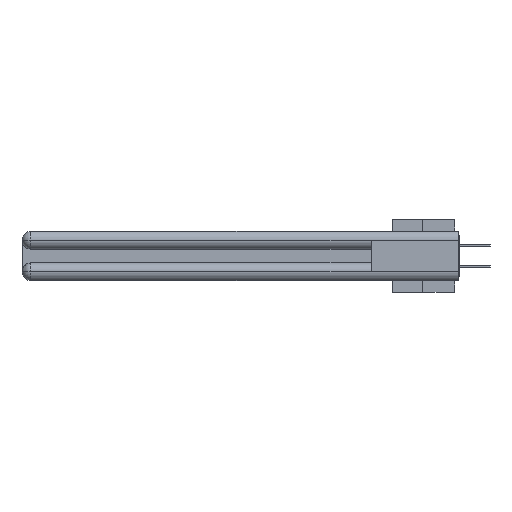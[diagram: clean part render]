
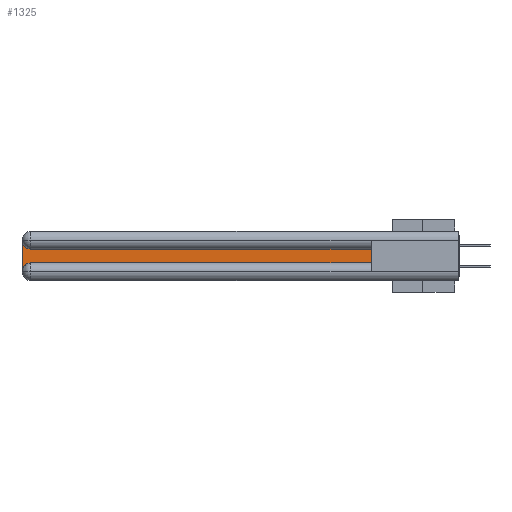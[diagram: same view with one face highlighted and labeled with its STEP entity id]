
A CAD part, left-side view. The second image highlights one B-rep face of the part: STEP entity #1325.
In plain terms, the highlighted planar face has unit normal (-1, 0, 0).
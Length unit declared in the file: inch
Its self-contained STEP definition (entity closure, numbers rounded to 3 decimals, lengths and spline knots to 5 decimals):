
#74 = VECTOR ( 'NONE', #16724, 39.37008 ) ;
#1325 = ADVANCED_FACE ( 'NONE', ( #25276 ), #7917, .F. ) ;
#1981 = LINE ( 'NONE', #8836, #11618 ) ;
#2189 = CARTESIAN_POINT ( 'NONE',  ( 0.075, 3., -0.1225 ) ) ;
#2423 = VECTOR ( 'NONE', #4829, 39.37008 ) ;
#2667 = EDGE_CURVE ( 'NONE', #15542, #8609, #1981, .T. ) ;
#4596 = CARTESIAN_POINT ( 'NONE',  ( 0.075, 3., -0.2775 ) ) ;
#4829 = DIRECTION ( 'NONE',  ( 0., 0., -1. ) ) ;
#6601 = EDGE_CURVE ( 'NONE', #27151, #16936, #23314, .T. ) ;
#7165 = DIRECTION ( 'NONE',  ( 0., 0., -1. ) ) ;
#7917 = PLANE ( 'NONE',  #29174 ) ;
#8261 = CARTESIAN_POINT ( 'NONE',  ( 0.075, 2.94, -0.1225 ) ) ;
#8609 = VERTEX_POINT ( 'NONE', #13999 ) ;
#8827 = VERTEX_POINT ( 'NONE', #4596 ) ;
#8836 = CARTESIAN_POINT ( 'NONE',  ( 0.075, 0.6, -0.2175 ) ) ;
#9289 = EDGE_CURVE ( 'NONE', #8609, #27151, #15545, .T. ) ;
#10502 = EDGE_CURVE ( 'NONE', #8827, #15542, #25737, .T. ) ;
#10585 = CARTESIAN_POINT ( 'NONE',  ( 0.075, 0.6, -0.1225 ) ) ;
#11618 = VECTOR ( 'NONE', #22608, 39.37008 ) ;
#12126 = EDGE_CURVE ( 'NONE', #16936, #31882, #32692, .T. ) ;
#13279 = ORIENTED_EDGE ( 'NONE', *, *, #10502, .T. ) ;
#13380 = DIRECTION ( 'NONE',  ( 0., 0., 1. ) ) ;
#13833 = LINE ( 'NONE', #34744, #2423 ) ;
#13999 = CARTESIAN_POINT ( 'NONE',  ( 0.075, 0.6, -0.2175 ) ) ;
#14164 = EDGE_CURVE ( 'NONE', #31882, #8827, #13833, .T. ) ;
#15086 = AXIS2_PLACEMENT_3D ( 'NONE', #36253, #19456, #19337 ) ;
#15542 = VERTEX_POINT ( 'NONE', #25339 ) ;
#15545 = LINE ( 'NONE', #21835, #26046 ) ;
#16284 = DIRECTION ( 'NONE',  ( 0., 0., -1. ) ) ;
#16724 = DIRECTION ( 'NONE',  ( 0., 1., 0. ) ) ;
#16936 = VERTEX_POINT ( 'NONE', #8261 ) ;
#18178 = ORIENTED_EDGE ( 'NONE', *, *, #12126, .T. ) ;
#19015 = ORIENTED_EDGE ( 'NONE', *, *, #14164, .T. ) ;
#19337 = DIRECTION ( 'NONE',  ( 0., 0., -1. ) ) ;
#19456 = DIRECTION ( 'NONE',  ( 1., 0., 0. ) ) ;
#19553 = ORIENTED_EDGE ( 'NONE', *, *, #6601, .T. ) ;
#19980 = AXIS2_PLACEMENT_3D ( 'NONE', #27188, #24442, #7165 ) ;
#21835 = CARTESIAN_POINT ( 'NONE',  ( 0.075, 0.6, -0.2175 ) ) ;
#22608 = DIRECTION ( 'NONE',  ( 0., -1., 0. ) ) ;
#23314 = LINE ( 'NONE', #33125, #74 ) ;
#24442 = DIRECTION ( 'NONE',  ( 1., 0., 0. ) ) ;
#25039 = CARTESIAN_POINT ( 'NONE',  ( 0.075, 3., -0.0625 ) ) ;
#25276 = FACE_OUTER_BOUND ( 'NONE', #32048, .T. ) ;
#25339 = CARTESIAN_POINT ( 'NONE',  ( 0.075, 2.94, -0.2175 ) ) ;
#25737 = CIRCLE ( 'NONE', #19980, 0.06 ) ;
#26046 = VECTOR ( 'NONE', #13380, 39.37008 ) ;
#27151 = VERTEX_POINT ( 'NONE', #10585 ) ;
#27188 = CARTESIAN_POINT ( 'NONE',  ( 0.075, 2.94, -0.2775 ) ) ;
#28441 = ORIENTED_EDGE ( 'NONE', *, *, #9289, .T. ) ;
#29174 = AXIS2_PLACEMENT_3D ( 'NONE', #2189, #33187, #16284 ) ;
#31112 = ORIENTED_EDGE ( 'NONE', *, *, #2667, .T. ) ;
#31882 = VERTEX_POINT ( 'NONE', #25039 ) ;
#32048 = EDGE_LOOP ( 'NONE', ( #19553, #18178, #19015, #13279, #31112, #28441 ) ) ;
#32692 = CIRCLE ( 'NONE', #15086, 0.06 ) ;
#33125 = CARTESIAN_POINT ( 'NONE',  ( 0.075, 0.6, -0.1225 ) ) ;
#33187 = DIRECTION ( 'NONE',  ( 1., 0., 0. ) ) ;
#34744 = CARTESIAN_POINT ( 'NONE',  ( 0.075, 3., -0.2175 ) ) ;
#36253 = CARTESIAN_POINT ( 'NONE',  ( 0.075, 2.94, -0.0625 ) ) ;
